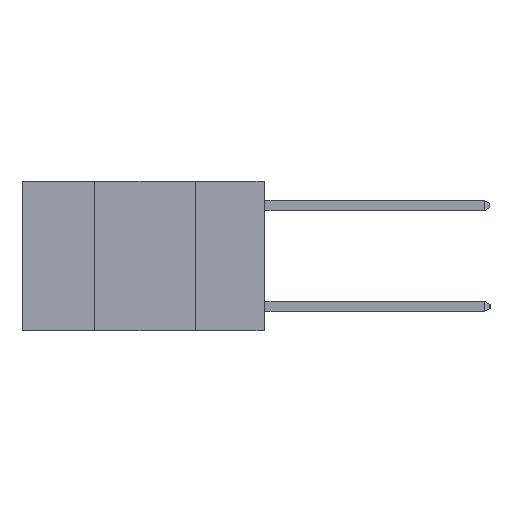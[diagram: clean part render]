
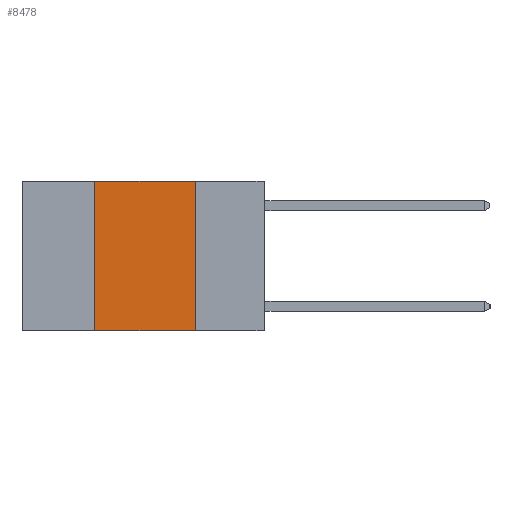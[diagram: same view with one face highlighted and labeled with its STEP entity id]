
A CAD part, left-side view. The second image highlights one B-rep face of the part: STEP entity #8478.
In plain terms, the highlighted planar face has unit normal (-1, 0, 0).
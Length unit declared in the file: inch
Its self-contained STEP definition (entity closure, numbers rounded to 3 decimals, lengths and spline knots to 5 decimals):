
#442 = EDGE_LOOP ( 'NONE', ( #6417, #2560, #4878, #966 ) ) ;
#486 = EDGE_CURVE ( 'NONE', #7804, #8825, #7856, .T. ) ;
#702 = CARTESIAN_POINT ( 'NONE',  ( 0., 0.17, 0. ) ) ;
#751 = DIRECTION ( 'NONE',  ( 0., 0., -1. ) ) ;
#966 = ORIENTED_EDGE ( 'NONE', *, *, #9777, .T. ) ;
#1798 = CARTESIAN_POINT ( 'NONE',  ( 0., 0.42, 0. ) ) ;
#2171 = CARTESIAN_POINT ( 'NONE',  ( 0., 0.17, 0. ) ) ;
#2279 = CARTESIAN_POINT ( 'NONE',  ( 0., 0.6, 0. ) ) ;
#2419 = VECTOR ( 'NONE', #3685, 39.37008 ) ;
#2560 = ORIENTED_EDGE ( 'NONE', *, *, #6283, .F. ) ;
#3131 = VECTOR ( 'NONE', #3351, 39.37008 ) ;
#3351 = DIRECTION ( 'NONE',  ( 0., -1., 0. ) ) ;
#3685 = DIRECTION ( 'NONE',  ( 0., -1., 0. ) ) ;
#3828 = VECTOR ( 'NONE', #8243, 39.37008 ) ;
#3830 = PLANE ( 'NONE',  #4860 ) ;
#4196 = DIRECTION ( 'NONE',  ( 0., 0., 1. ) ) ;
#4860 = AXIS2_PLACEMENT_3D ( 'NONE', #2279, #5410, #751 ) ;
#4878 = ORIENTED_EDGE ( 'NONE', *, *, #8738, .F. ) ;
#5119 = FACE_OUTER_BOUND ( 'NONE', #442, .T. ) ;
#5410 = DIRECTION ( 'NONE',  ( 1., 0., 0. ) ) ;
#5877 = CARTESIAN_POINT ( 'NONE',  ( 0., 0.42, -0.37 ) ) ;
#6283 = EDGE_CURVE ( 'NONE', #7865, #7804, #9200, .T. ) ;
#6406 = CARTESIAN_POINT ( 'NONE',  ( 0., 0.6, 0. ) ) ;
#6417 = ORIENTED_EDGE ( 'NONE', *, *, #486, .F. ) ;
#6525 = LINE ( 'NONE', #8229, #2419 ) ;
#7272 = CARTESIAN_POINT ( 'NONE',  ( 0., 0.17, -0.37 ) ) ;
#7804 = VERTEX_POINT ( 'NONE', #702 ) ;
#7856 = LINE ( 'NONE', #2171, #3828 ) ;
#7865 = VERTEX_POINT ( 'NONE', #9960 ) ;
#8229 = CARTESIAN_POINT ( 'NONE',  ( 0., 0.6, -0.37 ) ) ;
#8243 = DIRECTION ( 'NONE',  ( 0., 0., -1. ) ) ;
#8478 = ADVANCED_FACE ( 'NONE', ( #5119 ), #3830, .F. ) ;
#8738 = EDGE_CURVE ( 'NONE', #9689, #7865, #9498, .T. ) ;
#8825 = VERTEX_POINT ( 'NONE', #7272 ) ;
#9019 = VECTOR ( 'NONE', #4196, 39.37008 ) ;
#9200 = LINE ( 'NONE', #6406, #3131 ) ;
#9498 = LINE ( 'NONE', #1798, #9019 ) ;
#9689 = VERTEX_POINT ( 'NONE', #5877 ) ;
#9777 = EDGE_CURVE ( 'NONE', #9689, #8825, #6525, .T. ) ;
#9960 = CARTESIAN_POINT ( 'NONE',  ( 0., 0.42, 0. ) ) ;
